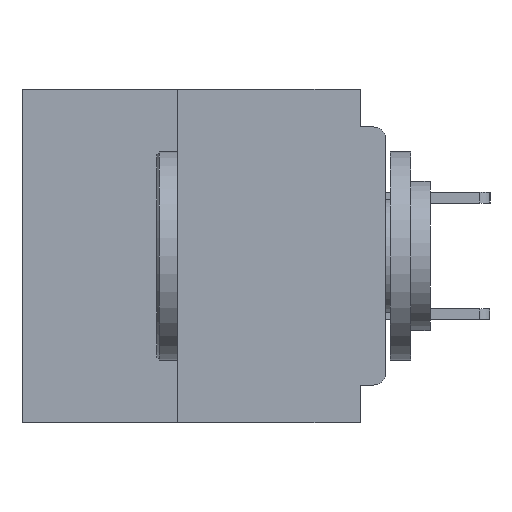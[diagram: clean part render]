
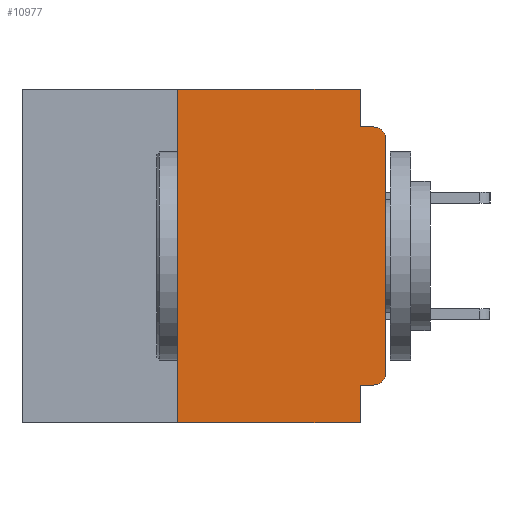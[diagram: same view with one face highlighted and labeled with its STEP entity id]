
A CAD part, left-side view. The second image highlights one B-rep face of the part: STEP entity #10977.
In plain terms, the highlighted planar face has unit normal (-1, 0, 0).
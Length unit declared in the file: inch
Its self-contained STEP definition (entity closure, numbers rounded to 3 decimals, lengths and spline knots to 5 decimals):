
#99 = DIRECTION ( 'NONE',  ( 0., 0., 1. ) ) ;
#363 = CARTESIAN_POINT ( 'NONE',  ( 0., 0.25, -0.4 ) ) ;
#604 = LINE ( 'NONE', #1499, #33405 ) ;
#814 = VERTEX_POINT ( 'NONE', #33990 ) ;
#1107 = FACE_OUTER_BOUND ( 'NONE', #24818, .T. ) ;
#1164 = EDGE_CURVE ( 'NONE', #38113, #28125, #13495, .T. ) ;
#1276 = CARTESIAN_POINT ( 'NONE',  ( 0., 0.437, -0.4 ) ) ;
#1499 = CARTESIAN_POINT ( 'NONE',  ( 0., 0.031, 0. ) ) ;
#1605 = CARTESIAN_POINT ( 'NONE',  ( 0., 0.031, -0.4 ) ) ;
#1709 = EDGE_CURVE ( 'NONE', #28125, #19270, #36806, .T. ) ;
#2287 = ORIENTED_EDGE ( 'NONE', *, *, #23262, .F. ) ;
#2831 = ORIENTED_EDGE ( 'NONE', *, *, #1709, .F. ) ;
#3583 = CARTESIAN_POINT ( 'NONE',  ( 0., 0.015, -0.34 ) ) ;
#3803 = DIRECTION ( 'NONE',  ( 0., -1., 0. ) ) ;
#3993 = VECTOR ( 'NONE', #35025, 39.37008 ) ;
#4359 = CARTESIAN_POINT ( 'NONE',  ( 0., 0., -0.355 ) ) ;
#4486 = DIRECTION ( 'NONE',  ( 0., -1., 0. ) ) ;
#4600 = CARTESIAN_POINT ( 'NONE',  ( 0., 0.031, -0.4 ) ) ;
#4816 = DIRECTION ( 'NONE',  ( 0., 0., -1. ) ) ;
#5914 = CARTESIAN_POINT ( 'NONE',  ( 0., 0., -0.34 ) ) ;
#5930 = VECTOR ( 'NONE', #3803, 39.37008 ) ;
#6065 = VECTOR ( 'NONE', #99, 39.37008 ) ;
#6712 = VERTEX_POINT ( 'NONE', #36734 ) ;
#6816 = DIRECTION ( 'NONE',  ( 0., 0., -1. ) ) ;
#7564 = DIRECTION ( 'NONE',  ( -1., 0., 0. ) ) ;
#8472 = DIRECTION ( 'NONE',  ( 0., 0., -1. ) ) ;
#9170 = ORIENTED_EDGE ( 'NONE', *, *, #26523, .F. ) ;
#10977 = ADVANCED_FACE ( 'NONE', ( #1107 ), #21122, .F. ) ;
#11570 = VECTOR ( 'NONE', #36069, 39.37008 ) ;
#12320 = VECTOR ( 'NONE', #29792, 39.37008 ) ;
#12440 = AXIS2_PLACEMENT_3D ( 'NONE', #26593, #7564, #29782 ) ;
#13495 = LINE ( 'NONE', #363, #6065 ) ;
#13713 = ORIENTED_EDGE ( 'NONE', *, *, #39951, .T. ) ;
#14292 = AXIS2_PLACEMENT_3D ( 'NONE', #3583, #25849, #6816 ) ;
#14551 = ORIENTED_EDGE ( 'NONE', *, *, #1164, .F. ) ;
#15496 = VERTEX_POINT ( 'NONE', #37470 ) ;
#17082 = CARTESIAN_POINT ( 'NONE',  ( 0., 0., 0. ) ) ;
#18679 = CARTESIAN_POINT ( 'NONE',  ( 0., 0.031, 0. ) ) ;
#19270 = VERTEX_POINT ( 'NONE', #18679 ) ;
#20048 = EDGE_CURVE ( 'NONE', #814, #34282, #27316, .T. ) ;
#20559 = DIRECTION ( 'NONE',  ( 0., 0., -1. ) ) ;
#20864 = EDGE_CURVE ( 'NONE', #814, #15496, #29237, .T. ) ;
#21122 = PLANE ( 'NONE',  #24252 ) ;
#21521 = EDGE_CURVE ( 'NONE', #32512, #6712, #34303, .T. ) ;
#22152 = LINE ( 'NONE', #1276, #37997 ) ;
#22688 = ORIENTED_EDGE ( 'NONE', *, *, #20048, .T. ) ;
#23033 = VECTOR ( 'NONE', #4816, 39.37008 ) ;
#23040 = CARTESIAN_POINT ( 'NONE',  ( 0., 0.031, -0.045 ) ) ;
#23262 = EDGE_CURVE ( 'NONE', #30496, #6712, #39656, .T. ) ;
#24252 = AXIS2_PLACEMENT_3D ( 'NONE', #24316, #27478, #8472 ) ;
#24316 = CARTESIAN_POINT ( 'NONE',  ( 0., 0.437, 0. ) ) ;
#24818 = EDGE_LOOP ( 'NONE', ( #13713, #29880, #2287, #40802, #2831, #14551, #31492, #9170, #40138, #22688 ) ) ;
#25304 = EDGE_CURVE ( 'NONE', #38113, #32828, #22152, .T. ) ;
#25849 = DIRECTION ( 'NONE',  ( -1., 0., 0. ) ) ;
#26059 = CARTESIAN_POINT ( 'NONE',  ( 0., 0., -0.045 ) ) ;
#26523 = EDGE_CURVE ( 'NONE', #15496, #32828, #31449, .T. ) ;
#26593 = CARTESIAN_POINT ( 'NONE',  ( 0., 0.015, -0.06 ) ) ;
#27042 = CARTESIAN_POINT ( 'NONE',  ( 0., 0., -0.06 ) ) ;
#27316 = CIRCLE ( 'NONE', #14292, 0.015 ) ;
#27478 = DIRECTION ( 'NONE',  ( 1., 0., 0. ) ) ;
#28125 = VERTEX_POINT ( 'NONE', #39985 ) ;
#28469 = LINE ( 'NONE', #17082, #11570 ) ;
#29237 = LINE ( 'NONE', #4359, #12320 ) ;
#29782 = DIRECTION ( 'NONE',  ( 0., 0., -1. ) ) ;
#29792 = DIRECTION ( 'NONE',  ( 0., 1., 0. ) ) ;
#29880 = ORIENTED_EDGE ( 'NONE', *, *, #21521, .T. ) ;
#30008 = CARTESIAN_POINT ( 'NONE',  ( 0., 0.25, -0.4 ) ) ;
#30496 = VERTEX_POINT ( 'NONE', #23040 ) ;
#31449 = LINE ( 'NONE', #1605, #23033 ) ;
#31492 = ORIENTED_EDGE ( 'NONE', *, *, #25304, .T. ) ;
#31934 = EDGE_CURVE ( 'NONE', #19270, #30496, #604, .T. ) ;
#32512 = VERTEX_POINT ( 'NONE', #27042 ) ;
#32828 = VERTEX_POINT ( 'NONE', #4600 ) ;
#33405 = VECTOR ( 'NONE', #20559, 39.37008 ) ;
#33990 = CARTESIAN_POINT ( 'NONE',  ( 0., 0.015, -0.355 ) ) ;
#34282 = VERTEX_POINT ( 'NONE', #5914 ) ;
#34303 = CIRCLE ( 'NONE', #12440, 0.015 ) ;
#34900 = CARTESIAN_POINT ( 'NONE',  ( 0., 0.437, 0. ) ) ;
#35025 = DIRECTION ( 'NONE',  ( 0., -1., 0. ) ) ;
#36069 = DIRECTION ( 'NONE',  ( 0., 0., 1. ) ) ;
#36734 = CARTESIAN_POINT ( 'NONE',  ( 0., 0.015, -0.045 ) ) ;
#36806 = LINE ( 'NONE', #34900, #3993 ) ;
#37470 = CARTESIAN_POINT ( 'NONE',  ( 0., 0.031, -0.355 ) ) ;
#37997 = VECTOR ( 'NONE', #4486, 39.37008 ) ;
#38113 = VERTEX_POINT ( 'NONE', #30008 ) ;
#39656 = LINE ( 'NONE', #26059, #5930 ) ;
#39951 = EDGE_CURVE ( 'NONE', #34282, #32512, #28469, .T. ) ;
#39985 = CARTESIAN_POINT ( 'NONE',  ( 0., 0.25, 0. ) ) ;
#40138 = ORIENTED_EDGE ( 'NONE', *, *, #20864, .F. ) ;
#40802 = ORIENTED_EDGE ( 'NONE', *, *, #31934, .F. ) ;
